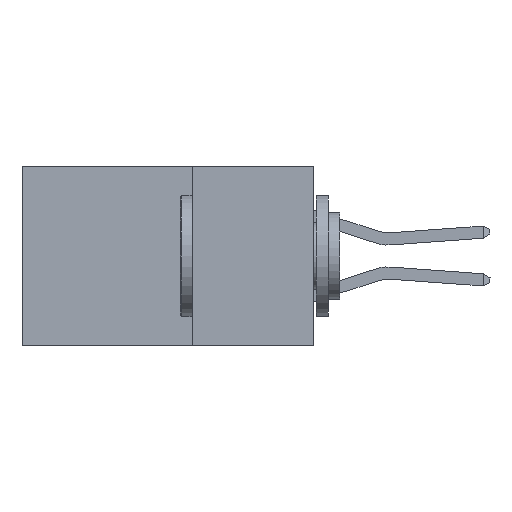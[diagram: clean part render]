
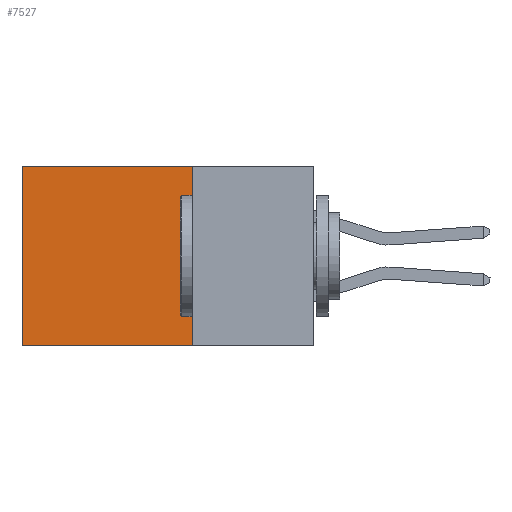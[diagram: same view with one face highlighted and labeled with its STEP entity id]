
A CAD part, left-side view. The second image highlights one B-rep face of the part: STEP entity #7527.
In plain terms, the highlighted planar face has unit normal (-1, 0, 0).
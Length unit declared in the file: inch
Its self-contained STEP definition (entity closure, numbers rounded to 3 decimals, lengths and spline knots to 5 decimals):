
#2480 = VERTEX_POINT ( 'NONE', #17977 ) ;
#6882 = VECTOR ( 'NONE', #13616, 39.37008 ) ;
#7527 = ADVANCED_FACE ( 'NONE', ( #38159 ), #24443, .F. ) ;
#8362 = VERTEX_POINT ( 'NONE', #21922 ) ;
#10113 = LINE ( 'NONE', #33202, #6882 ) ;
#10548 = CARTESIAN_POINT ( 'NONE',  ( 0.2875, 0.6, 0. ) ) ;
#11841 = CARTESIAN_POINT ( 'NONE',  ( 0.2875, 0.6, 0. ) ) ;
#12795 = CARTESIAN_POINT ( 'NONE',  ( 0.2875, 0.25, 0. ) ) ;
#13616 = DIRECTION ( 'NONE',  ( 0., 0., -1. ) ) ;
#13771 = ORIENTED_EDGE ( 'NONE', *, *, #36639, .F. ) ;
#15816 = CARTESIAN_POINT ( 'NONE',  ( 0.2875, 0.25, -0.37 ) ) ;
#15956 = EDGE_LOOP ( 'NONE', ( #24529, #13771, #26980, #25879 ) ) ;
#16096 = LINE ( 'NONE', #15816, #29056 ) ;
#17977 = CARTESIAN_POINT ( 'NONE',  ( 0.2875, 0.6, -0.37 ) ) ;
#19073 = DIRECTION ( 'NONE',  ( 0., 1., 0. ) ) ;
#19830 = EDGE_CURVE ( 'NONE', #8362, #27237, #29843, .T. ) ;
#21196 = DIRECTION ( 'NONE',  ( 0., 0., -1. ) ) ;
#21314 = LINE ( 'NONE', #10548, #21805 ) ;
#21805 = VECTOR ( 'NONE', #31162, 39.37008 ) ;
#21922 = CARTESIAN_POINT ( 'NONE',  ( 0.2875, 0.25, 0. ) ) ;
#22010 = DIRECTION ( 'NONE',  ( 0., 1., 0. ) ) ;
#22938 = VECTOR ( 'NONE', #22010, 39.37008 ) ;
#23178 = EDGE_CURVE ( 'NONE', #27237, #2480, #21314, .T. ) ;
#24443 = PLANE ( 'NONE',  #36840 ) ;
#24529 = ORIENTED_EDGE ( 'NONE', *, *, #23178, .T. ) ;
#25220 = CARTESIAN_POINT ( 'NONE',  ( 0.2875, 0.25, -0.37 ) ) ;
#25879 = ORIENTED_EDGE ( 'NONE', *, *, #19830, .T. ) ;
#26980 = ORIENTED_EDGE ( 'NONE', *, *, #31526, .F. ) ;
#27237 = VERTEX_POINT ( 'NONE', #11841 ) ;
#29036 = VERTEX_POINT ( 'NONE', #25220 ) ;
#29056 = VECTOR ( 'NONE', #19073, 39.37008 ) ;
#29843 = LINE ( 'NONE', #36072, #22938 ) ;
#31162 = DIRECTION ( 'NONE',  ( 0., 0., -1. ) ) ;
#31526 = EDGE_CURVE ( 'NONE', #8362, #29036, #10113, .T. ) ;
#33202 = CARTESIAN_POINT ( 'NONE',  ( 0.2875, 0.25, 0. ) ) ;
#36072 = CARTESIAN_POINT ( 'NONE',  ( 0.2875, 0.25, 0. ) ) ;
#36419 = DIRECTION ( 'NONE',  ( 1., 0., 0. ) ) ;
#36639 = EDGE_CURVE ( 'NONE', #29036, #2480, #16096, .T. ) ;
#36840 = AXIS2_PLACEMENT_3D ( 'NONE', #12795, #36419, #21196 ) ;
#38159 = FACE_OUTER_BOUND ( 'NONE', #15956, .T. ) ;
